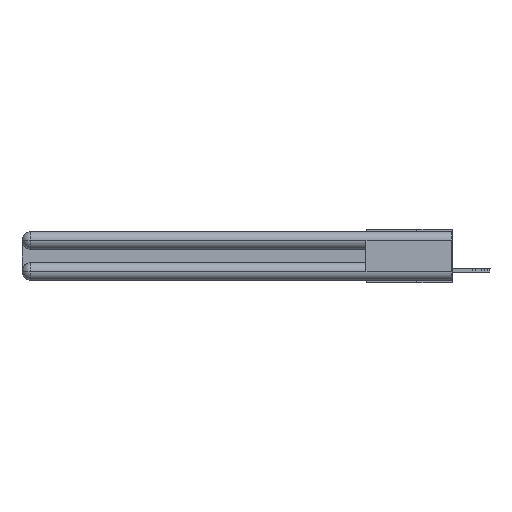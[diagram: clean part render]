
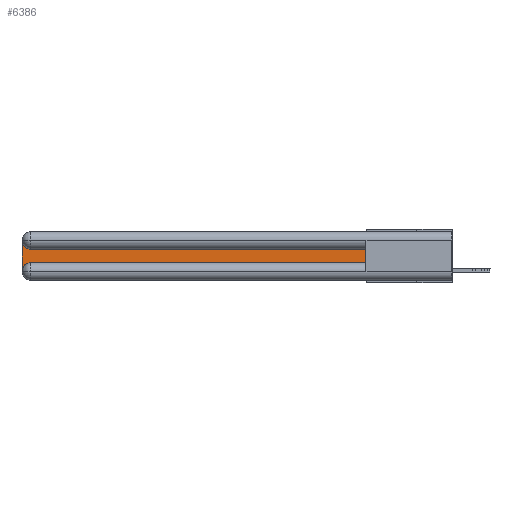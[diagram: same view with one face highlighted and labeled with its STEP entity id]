
A CAD part, left-side view. The second image highlights one B-rep face of the part: STEP entity #6386.
In plain terms, the highlighted planar face has unit normal (-1, 0, 0).
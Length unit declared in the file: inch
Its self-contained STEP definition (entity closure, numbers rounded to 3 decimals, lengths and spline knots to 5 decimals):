
#414 = DIRECTION ( 'NONE',  ( 0., 0., -1. ) ) ;
#600 = CARTESIAN_POINT ( 'NONE',  ( 0.075, 0.6, -0.2175 ) ) ;
#683 = VERTEX_POINT ( 'NONE', #25907 ) ;
#692 = DIRECTION ( 'NONE',  ( 0., -1., 0. ) ) ;
#1765 = VERTEX_POINT ( 'NONE', #27917 ) ;
#3811 = DIRECTION ( 'NONE',  ( 1., 0., 0. ) ) ;
#4648 = CARTESIAN_POINT ( 'NONE',  ( 0.075, 2.94, -0.2175 ) ) ;
#4919 = EDGE_CURVE ( 'NONE', #5824, #1765, #18934, .T. ) ;
#5824 = VERTEX_POINT ( 'NONE', #24339 ) ;
#6339 = DIRECTION ( 'NONE',  ( 1., 0., 0. ) ) ;
#6386 = ADVANCED_FACE ( 'NONE', ( #11160 ), #15423, .F. ) ;
#7477 = VERTEX_POINT ( 'NONE', #22559 ) ;
#7732 = VECTOR ( 'NONE', #414, 39.37008 ) ;
#7762 = EDGE_CURVE ( 'NONE', #23873, #5824, #27832, .T. ) ;
#8043 = VECTOR ( 'NONE', #9093, 39.37008 ) ;
#8781 = CARTESIAN_POINT ( 'NONE',  ( 0.075, 3., -0.1225 ) ) ;
#8913 = AXIS2_PLACEMENT_3D ( 'NONE', #19295, #6339, #23898 ) ;
#9093 = DIRECTION ( 'NONE',  ( 0., 1., 0. ) ) ;
#9191 = CARTESIAN_POINT ( 'NONE',  ( 0.075, 0.6, -0.1225 ) ) ;
#9210 = CARTESIAN_POINT ( 'NONE',  ( 0.075, 0.6, -0.1225 ) ) ;
#11160 = FACE_OUTER_BOUND ( 'NONE', #17633, .T. ) ;
#12475 = EDGE_CURVE ( 'NONE', #7477, #23873, #14721, .T. ) ;
#12560 = CARTESIAN_POINT ( 'NONE',  ( 0.075, 2.94, -0.2775 ) ) ;
#12769 = EDGE_CURVE ( 'NONE', #683, #15185, #15021, .T. ) ;
#13201 = LINE ( 'NONE', #26393, #7732 ) ;
#13438 = ORIENTED_EDGE ( 'NONE', *, *, #7762, .T. ) ;
#14721 = LINE ( 'NONE', #24791, #17806 ) ;
#15021 = CIRCLE ( 'NONE', #25548, 0.06 ) ;
#15185 = VERTEX_POINT ( 'NONE', #4648 ) ;
#15423 = PLANE ( 'NONE',  #20846 ) ;
#16589 = VECTOR ( 'NONE', #692, 39.37008 ) ;
#16728 = EDGE_CURVE ( 'NONE', #1765, #683, #13201, .T. ) ;
#17050 = DIRECTION ( 'NONE',  ( 0., 0., -1. ) ) ;
#17633 = EDGE_LOOP ( 'NONE', ( #13438, #19006, #25524, #18369, #27067, #19131 ) ) ;
#17806 = VECTOR ( 'NONE', #20280, 39.37008 ) ;
#18369 = ORIENTED_EDGE ( 'NONE', *, *, #12769, .T. ) ;
#18934 = CIRCLE ( 'NONE', #8913, 0.06 ) ;
#19006 = ORIENTED_EDGE ( 'NONE', *, *, #4919, .T. ) ;
#19131 = ORIENTED_EDGE ( 'NONE', *, *, #12475, .T. ) ;
#19295 = CARTESIAN_POINT ( 'NONE',  ( 0.075, 2.94, -0.0625 ) ) ;
#20280 = DIRECTION ( 'NONE',  ( 0., 0., 1. ) ) ;
#20846 = AXIS2_PLACEMENT_3D ( 'NONE', #8781, #23960, #24242 ) ;
#22559 = CARTESIAN_POINT ( 'NONE',  ( 0.075, 0.6, -0.2175 ) ) ;
#23873 = VERTEX_POINT ( 'NONE', #9210 ) ;
#23898 = DIRECTION ( 'NONE',  ( 0., 0., -1. ) ) ;
#23960 = DIRECTION ( 'NONE',  ( 1., 0., 0. ) ) ;
#24242 = DIRECTION ( 'NONE',  ( 0., 0., -1. ) ) ;
#24339 = CARTESIAN_POINT ( 'NONE',  ( 0.075, 2.94, -0.1225 ) ) ;
#24791 = CARTESIAN_POINT ( 'NONE',  ( 0.075, 0.6, -0.2175 ) ) ;
#24821 = LINE ( 'NONE', #600, #16589 ) ;
#25524 = ORIENTED_EDGE ( 'NONE', *, *, #16728, .T. ) ;
#25548 = AXIS2_PLACEMENT_3D ( 'NONE', #12560, #3811, #17050 ) ;
#25907 = CARTESIAN_POINT ( 'NONE',  ( 0.075, 3., -0.2775 ) ) ;
#26392 = EDGE_CURVE ( 'NONE', #15185, #7477, #24821, .T. ) ;
#26393 = CARTESIAN_POINT ( 'NONE',  ( 0.075, 3., -0.2175 ) ) ;
#27067 = ORIENTED_EDGE ( 'NONE', *, *, #26392, .T. ) ;
#27832 = LINE ( 'NONE', #9191, #8043 ) ;
#27917 = CARTESIAN_POINT ( 'NONE',  ( 0.075, 3., -0.0625 ) ) ;
